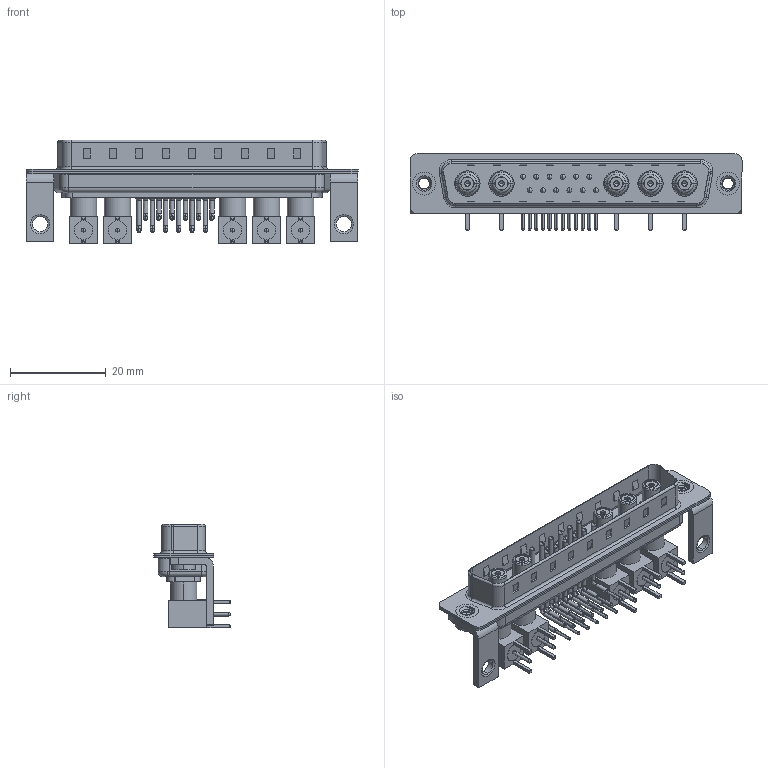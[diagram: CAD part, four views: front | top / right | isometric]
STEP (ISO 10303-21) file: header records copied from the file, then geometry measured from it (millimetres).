
FILE_DESCRIPTION (( 'STEP AP203' ), '1' );
FILE_NAME ('629-17W5240-5TC.STEP', '2022-05-14T23:48:25', ( '' ), ( '' ), 'SwSTEP 2.0', 'SolidWorks 2020', '' );
FILE_SCHEMA (( 'CONFIG_CONTROL_DESIGN' ));
Length unit declared in the file: millimetre
Products named in the file (20): 629Combo Shell Rear_37 Contacts; Socket_RA; Co-Ax Jack Assy_RA; 629Combo Contact Row 2; Insulator RA Pin; 629-17W5240-5TC; 629Combo Contact Row 1; 629Combo Stabilizer Bracket; 629Combo Housing_17W5; Locking Collar; Insulator Socket; RA Back Shell; Insulator Socket 2; 629Combo Shell Front_37 Contacts; Co-Ax Jack_RA PC Tail; 629Combo Threaded Rivet_2
Assembly tree (59 placements, depth 3):
  629-17W5240-5TC
    629Combo Housing_17W5
    629Combo Shell Rear_37 Contacts
    629Combo Shell Front_37 Contacts
    629Combo Threaded Rivet_2  x2
    629Combo Stabilizer Bracket  x2
    Co-Ax Jack Assy_RA
      Co-Ax Jack_RA PC Tail
      Insulator Socket
      Insulator Socket 2
      Locking Collar
      Socket_RA
      RA Back Shell
      Insulator RA Pin
    Co-Ax Jack Assy_RA
      Co-Ax Jack_RA PC Tail
      Insulator Socket
      Insulator Socket 2
      Locking Collar
      Socket_RA
      RA Back Shell
      Insulator RA Pin
    Co-Ax Jack Assy_RA
      Co-Ax Jack_RA PC Tail
      Insulator Socket
      Insulator Socket 2
      Locking Collar
      Socket_RA
      RA Back Shell
      Insulator RA Pin
    Co-Ax Jack Assy_RA
      Co-Ax Jack_RA PC Tail
      Insulator Socket
      Insulator Socket 2
      Locking Collar
      Socket_RA
      RA Back Shell
      Insulator RA Pin
    Co-Ax Jack Assy_RA
      Co-Ax Jack_RA PC Tail
      Insulator Socket
      Insulator Socket 2
      Locking Collar
      Socket_RA
      RA Back Shell
      Insulator RA Pin
    629Combo Contact Row 1  x6
    629Combo Contact Row 2  x6
Bounding box: 69.4 x 16 x 21.71 mm (x, y, z)
Volume: 5602.9 mm3; surface area: 14853.3 mm2
Topology: 54 solids, 54 shells, 2540 faces, 6642 edges, 4251 vertices
Faces by surface type: plane 1276, cylinder 932, cone 159, bspline 83, torus 80, sphere 10
Entity records: 31689 total; most frequent: CARTESIAN_POINT 6492, DIRECTION 4812, ORIENTED_EDGE 4430, EDGE_CURVE 2215, AXIS2_PLACEMENT_3D 1736, VERTEX_POINT 1425, LINE 1340, VECTOR 1340
